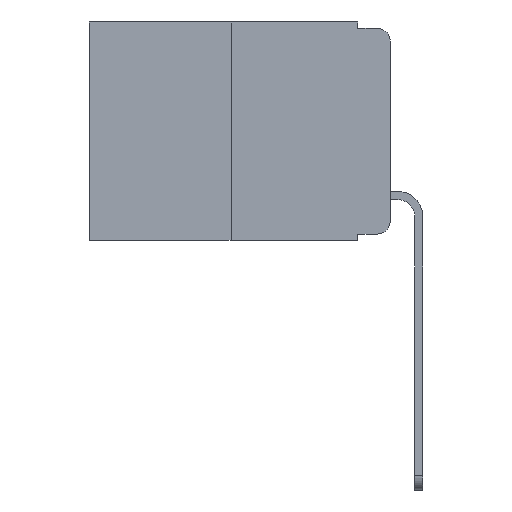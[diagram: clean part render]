
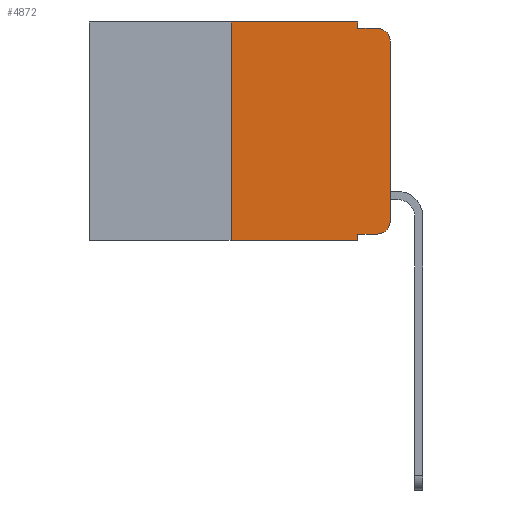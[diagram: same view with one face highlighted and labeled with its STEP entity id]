
A CAD part, left-side view. The second image highlights one B-rep face of the part: STEP entity #4872.
In plain terms, the highlighted planar face has unit normal (-1, 0, 0).
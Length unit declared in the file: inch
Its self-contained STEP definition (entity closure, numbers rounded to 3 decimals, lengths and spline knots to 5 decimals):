
#60 = ORIENTED_EDGE ( 'NONE', *, *, #9977, .F. ) ;
#115 = VERTEX_POINT ( 'NONE', #5872 ) ;
#791 = LINE ( 'NONE', #4332, #13077 ) ;
#954 = VERTEX_POINT ( 'NONE', #7866 ) ;
#1077 = DIRECTION ( 'NONE',  ( 1., 0., 0. ) ) ;
#1086 = VECTOR ( 'NONE', #2508, 39.37008 ) ;
#1328 = VERTEX_POINT ( 'NONE', #10840 ) ;
#1507 = CARTESIAN_POINT ( 'NONE',  ( 0., 0.473, -0.343 ) ) ;
#1722 = CARTESIAN_POINT ( 'NONE',  ( 0., 0.051, -0.01 ) ) ;
#1727 = VERTEX_POINT ( 'NONE', #11079 ) ;
#1895 = VECTOR ( 'NONE', #11448, 39.37008 ) ;
#1961 = DIRECTION ( 'NONE',  ( -1., 0., 0. ) ) ;
#2314 = ORIENTED_EDGE ( 'NONE', *, *, #12823, .T. ) ;
#2508 = DIRECTION ( 'NONE',  ( 0., 0., 1. ) ) ;
#2687 = ORIENTED_EDGE ( 'NONE', *, *, #13538, .T. ) ;
#2812 = AXIS2_PLACEMENT_3D ( 'NONE', #11096, #4145, #12179 ) ;
#2900 = VERTEX_POINT ( 'NONE', #9071 ) ;
#2913 = DIRECTION ( 'NONE',  ( 0., -1., 0. ) ) ;
#3056 = ORIENTED_EDGE ( 'NONE', *, *, #14660, .T. ) ;
#3241 = CARTESIAN_POINT ( 'NONE',  ( 0., 0.051, -0.333 ) ) ;
#4145 = DIRECTION ( 'NONE',  ( -1., 0., 0. ) ) ;
#4167 = LINE ( 'NONE', #8136, #7797 ) ;
#4332 = CARTESIAN_POINT ( 'NONE',  ( 0., 0.473, 0. ) ) ;
#4397 = DIRECTION ( 'NONE',  ( 0., -1., 0. ) ) ;
#4410 = VECTOR ( 'NONE', #2913, 39.37008 ) ;
#4527 = CARTESIAN_POINT ( 'NONE',  ( 0., 0.02, -0.01 ) ) ;
#4872 = ADVANCED_FACE ( 'NONE', ( #8036 ), #5075, .F. ) ;
#5075 = PLANE ( 'NONE',  #14169 ) ;
#5306 = EDGE_CURVE ( 'NONE', #2900, #1727, #791, .T. ) ;
#5371 = LINE ( 'NONE', #1722, #1895 ) ;
#5630 = CARTESIAN_POINT ( 'NONE',  ( 0., 0.051, -0.343 ) ) ;
#5872 = CARTESIAN_POINT ( 'NONE',  ( 0., 0., -0.313 ) ) ;
#6239 = CARTESIAN_POINT ( 'NONE',  ( 0., 0.051, -0.333 ) ) ;
#6244 = DIRECTION ( 'NONE',  ( 0., 0., -1. ) ) ;
#6306 = VECTOR ( 'NONE', #11068, 39.37008 ) ;
#6707 = VECTOR ( 'NONE', #9298, 39.37008 ) ;
#6764 = EDGE_LOOP ( 'NONE', ( #2687, #2314, #7911, #8069, #7824, #12544, #3056, #60, #8169, #12750 ) ) ;
#7466 = CARTESIAN_POINT ( 'NONE',  ( 0., 0.473, 0. ) ) ;
#7646 = LINE ( 'NONE', #1507, #4410 ) ;
#7797 = VECTOR ( 'NONE', #9267, 39.37008 ) ;
#7819 = CARTESIAN_POINT ( 'NONE',  ( 0., 0., -0.03 ) ) ;
#7824 = ORIENTED_EDGE ( 'NONE', *, *, #5306, .F. ) ;
#7866 = CARTESIAN_POINT ( 'NONE',  ( 0., 0.25, -0.343 ) ) ;
#7911 = ORIENTED_EDGE ( 'NONE', *, *, #12150, .F. ) ;
#8036 = FACE_OUTER_BOUND ( 'NONE', #6764, .T. ) ;
#8069 = ORIENTED_EDGE ( 'NONE', *, *, #11433, .F. ) ;
#8136 = CARTESIAN_POINT ( 'NONE',  ( 0., 0., 0. ) ) ;
#8169 = ORIENTED_EDGE ( 'NONE', *, *, #9253, .T. ) ;
#8491 = EDGE_CURVE ( 'NONE', #1328, #115, #11522, .T. ) ;
#8979 = VERTEX_POINT ( 'NONE', #7819 ) ;
#9071 = CARTESIAN_POINT ( 'NONE',  ( 0., 0.25, 0. ) ) ;
#9253 = EDGE_CURVE ( 'NONE', #10682, #1328, #12331, .T. ) ;
#9267 = DIRECTION ( 'NONE',  ( 0., 0., 1. ) ) ;
#9298 = DIRECTION ( 'NONE',  ( 0., -1., 0. ) ) ;
#9315 = AXIS2_PLACEMENT_3D ( 'NONE', #9359, #1961, #10457 ) ;
#9359 = CARTESIAN_POINT ( 'NONE',  ( 0., 0.02, -0.313 ) ) ;
#9422 = CARTESIAN_POINT ( 'NONE',  ( 0., 0.051, 0. ) ) ;
#9494 = VERTEX_POINT ( 'NONE', #13747 ) ;
#9977 = EDGE_CURVE ( 'NONE', #10682, #11089, #11989, .T. ) ;
#9986 = CARTESIAN_POINT ( 'NONE',  ( 0., 0.051, 0. ) ) ;
#10295 = VECTOR ( 'NONE', #13703, 39.37008 ) ;
#10457 = DIRECTION ( 'NONE',  ( 0., 0., -1. ) ) ;
#10485 = LINE ( 'NONE', #10861, #1086 ) ;
#10682 = VERTEX_POINT ( 'NONE', #6239 ) ;
#10696 = EDGE_CURVE ( 'NONE', #954, #2900, #10485, .T. ) ;
#10840 = CARTESIAN_POINT ( 'NONE',  ( 0., 0.02, -0.333 ) ) ;
#10861 = CARTESIAN_POINT ( 'NONE',  ( 0., 0.25, 0. ) ) ;
#11068 = DIRECTION ( 'NONE',  ( 0., 0., -1. ) ) ;
#11079 = CARTESIAN_POINT ( 'NONE',  ( 0., 0.051, 0. ) ) ;
#11089 = VERTEX_POINT ( 'NONE', #5630 ) ;
#11096 = CARTESIAN_POINT ( 'NONE',  ( 0., 0.02, -0.03 ) ) ;
#11217 = VERTEX_POINT ( 'NONE', #4527 ) ;
#11433 = EDGE_CURVE ( 'NONE', #1727, #9494, #13104, .T. ) ;
#11448 = DIRECTION ( 'NONE',  ( 0., -1., 0. ) ) ;
#11522 = CIRCLE ( 'NONE', #9315, 0.02 ) ;
#11599 = CIRCLE ( 'NONE', #2812, 0.02 ) ;
#11989 = LINE ( 'NONE', #9986, #6306 ) ;
#12150 = EDGE_CURVE ( 'NONE', #9494, #11217, #5371, .T. ) ;
#12179 = DIRECTION ( 'NONE',  ( 0., 0., -1. ) ) ;
#12331 = LINE ( 'NONE', #3241, #6707 ) ;
#12544 = ORIENTED_EDGE ( 'NONE', *, *, #10696, .F. ) ;
#12750 = ORIENTED_EDGE ( 'NONE', *, *, #8491, .T. ) ;
#12823 = EDGE_CURVE ( 'NONE', #8979, #11217, #11599, .T. ) ;
#13077 = VECTOR ( 'NONE', #4397, 39.37008 ) ;
#13104 = LINE ( 'NONE', #9422, #10295 ) ;
#13538 = EDGE_CURVE ( 'NONE', #115, #8979, #4167, .T. ) ;
#13703 = DIRECTION ( 'NONE',  ( 0., 0., -1. ) ) ;
#13747 = CARTESIAN_POINT ( 'NONE',  ( 0., 0.051, -0.01 ) ) ;
#14169 = AXIS2_PLACEMENT_3D ( 'NONE', #7466, #1077, #6244 ) ;
#14660 = EDGE_CURVE ( 'NONE', #954, #11089, #7646, .T. ) ;
